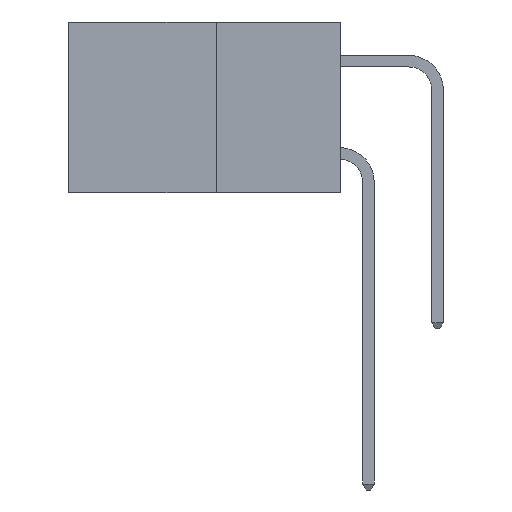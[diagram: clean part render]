
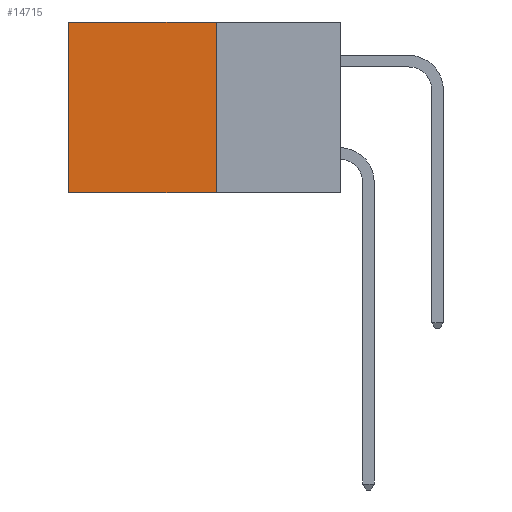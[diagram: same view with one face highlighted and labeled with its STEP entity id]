
A CAD part, left-side view. The second image highlights one B-rep face of the part: STEP entity #14715.
In plain terms, the highlighted planar face has unit normal (-1, 0, 0).
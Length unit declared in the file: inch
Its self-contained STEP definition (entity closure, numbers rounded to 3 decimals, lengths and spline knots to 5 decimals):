
#178 = DIRECTION ( 'NONE',  ( 0., 0., -1. ) ) ;
#278 = CARTESIAN_POINT ( 'NONE',  ( 0.277, 0.59, -0.37 ) ) ;
#794 = DIRECTION ( 'NONE',  ( 0., 0., -1. ) ) ;
#811 = VERTEX_POINT ( 'NONE', #278 ) ;
#1870 = VECTOR ( 'NONE', #18276, 39.37008 ) ;
#3508 = LINE ( 'NONE', #10588, #17278 ) ;
#3648 = VERTEX_POINT ( 'NONE', #10026 ) ;
#5007 = DIRECTION ( 'NONE',  ( 0., 1., 0. ) ) ;
#5362 = CARTESIAN_POINT ( 'NONE',  ( 0.277, 0.59, -0.37 ) ) ;
#8875 = LINE ( 'NONE', #17898, #28286 ) ;
#9092 = VERTEX_POINT ( 'NONE', #17609 ) ;
#9315 = CARTESIAN_POINT ( 'NONE',  ( 0.277, 0.59, 0. ) ) ;
#9380 = ORIENTED_EDGE ( 'NONE', *, *, #22019, .T. ) ;
#9657 = EDGE_LOOP ( 'NONE', ( #9380, #10156, #14112, #15529 ) ) ;
#9871 = EDGE_CURVE ( 'NONE', #3648, #811, #8875, .T. ) ;
#10026 = CARTESIAN_POINT ( 'NONE',  ( 0.277, 0.27, -0.37 ) ) ;
#10156 = ORIENTED_EDGE ( 'NONE', *, *, #9871, .F. ) ;
#10588 = CARTESIAN_POINT ( 'NONE',  ( 0.277, 0.27, 0. ) ) ;
#11179 = EDGE_CURVE ( 'NONE', #9092, #13537, #3508, .T. ) ;
#13537 = VERTEX_POINT ( 'NONE', #9315 ) ;
#14112 = ORIENTED_EDGE ( 'NONE', *, *, #25078, .F. ) ;
#14715 = ADVANCED_FACE ( 'NONE', ( #25312 ), #31207, .F. ) ;
#15449 = AXIS2_PLACEMENT_3D ( 'NONE', #18748, #16252, #794 ) ;
#15529 = ORIENTED_EDGE ( 'NONE', *, *, #11179, .T. ) ;
#16252 = DIRECTION ( 'NONE',  ( 1., 0., 0. ) ) ;
#16550 = LINE ( 'NONE', #5362, #23321 ) ;
#17278 = VECTOR ( 'NONE', #28272, 39.37008 ) ;
#17609 = CARTESIAN_POINT ( 'NONE',  ( 0.277, 0.27, 0. ) ) ;
#17898 = CARTESIAN_POINT ( 'NONE',  ( 0.277, 0.27, -0.37 ) ) ;
#18276 = DIRECTION ( 'NONE',  ( 0., 0., -1. ) ) ;
#18748 = CARTESIAN_POINT ( 'NONE',  ( 0.277, 0.27, -0.37 ) ) ;
#21604 = LINE ( 'NONE', #30629, #1870 ) ;
#22019 = EDGE_CURVE ( 'NONE', #13537, #811, #16550, .T. ) ;
#23321 = VECTOR ( 'NONE', #178, 39.37008 ) ;
#25078 = EDGE_CURVE ( 'NONE', #9092, #3648, #21604, .T. ) ;
#25312 = FACE_OUTER_BOUND ( 'NONE', #9657, .T. ) ;
#28272 = DIRECTION ( 'NONE',  ( 0., 1., 0. ) ) ;
#28286 = VECTOR ( 'NONE', #5007, 39.37008 ) ;
#30629 = CARTESIAN_POINT ( 'NONE',  ( 0.277, 0.27, -0.37 ) ) ;
#31207 = PLANE ( 'NONE',  #15449 ) ;
